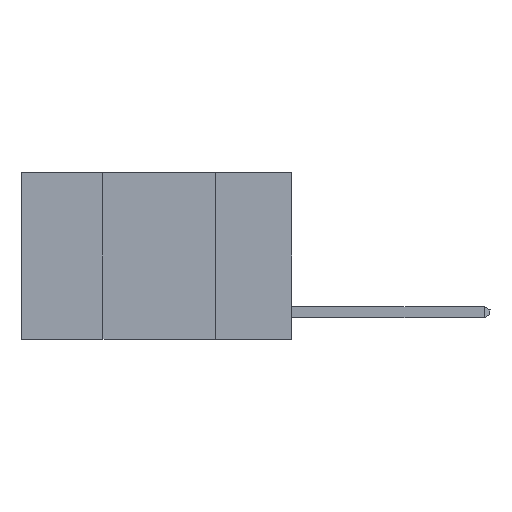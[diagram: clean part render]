
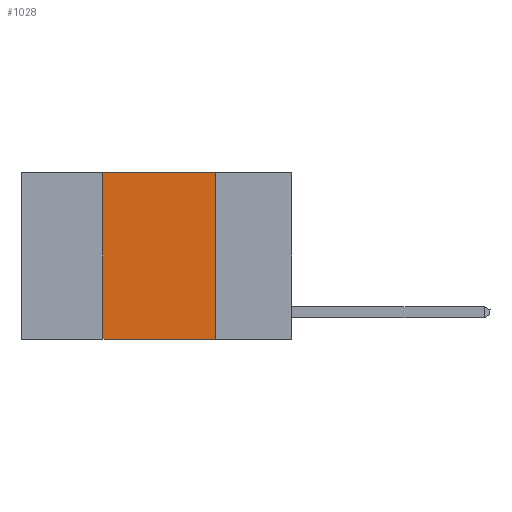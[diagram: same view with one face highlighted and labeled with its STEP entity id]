
A CAD part, left-side view. The second image highlights one B-rep face of the part: STEP entity #1028.
In plain terms, the highlighted planar face has unit normal (-1, 0, 0).
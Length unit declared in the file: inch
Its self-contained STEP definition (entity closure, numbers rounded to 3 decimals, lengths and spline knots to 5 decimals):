
#1028 = ADVANCED_FACE ( 'NONE', ( #15249 ), #13510, .F. ) ;
#2885 = CARTESIAN_POINT ( 'NONE',  ( 0., 0.17, 0. ) ) ;
#3431 = LINE ( 'NONE', #13747, #8251 ) ;
#3670 = VERTEX_POINT ( 'NONE', #6713 ) ;
#4139 = EDGE_CURVE ( 'NONE', #3670, #15752, #3431, .T. ) ;
#4483 = ORIENTED_EDGE ( 'NONE', *, *, #4139, .F. ) ;
#5009 = VECTOR ( 'NONE', #19134, 39.37008 ) ;
#6699 = CARTESIAN_POINT ( 'NONE',  ( 0., 0.6, -0.37 ) ) ;
#6713 = CARTESIAN_POINT ( 'NONE',  ( 0., 0.42, 0. ) ) ;
#7006 = ORIENTED_EDGE ( 'NONE', *, *, #11536, .T. ) ;
#7026 = LINE ( 'NONE', #15766, #8327 ) ;
#8251 = VECTOR ( 'NONE', #26389, 39.37008 ) ;
#8327 = VECTOR ( 'NONE', #21846, 39.37008 ) ;
#8535 = VECTOR ( 'NONE', #25374, 39.37008 ) ;
#10276 = VERTEX_POINT ( 'NONE', #21346 ) ;
#11498 = LINE ( 'NONE', #6699, #5009 ) ;
#11536 = EDGE_CURVE ( 'NONE', #10276, #22164, #11498, .T. ) ;
#11860 = EDGE_CURVE ( 'NONE', #15752, #22164, #19908, .T. ) ;
#13510 = PLANE ( 'NONE',  #16265 ) ;
#13747 = CARTESIAN_POINT ( 'NONE',  ( 0., 0.6, 0. ) ) ;
#14079 = DIRECTION ( 'NONE',  ( 0., 0., -1. ) ) ;
#14887 = CARTESIAN_POINT ( 'NONE',  ( 0., 0.17, -0.37 ) ) ;
#15249 = FACE_OUTER_BOUND ( 'NONE', #20489, .T. ) ;
#15752 = VERTEX_POINT ( 'NONE', #22078 ) ;
#15766 = CARTESIAN_POINT ( 'NONE',  ( 0., 0.42, 0. ) ) ;
#16265 = AXIS2_PLACEMENT_3D ( 'NONE', #19367, #24610, #14079 ) ;
#19134 = DIRECTION ( 'NONE',  ( 0., -1., 0. ) ) ;
#19367 = CARTESIAN_POINT ( 'NONE',  ( 0., 0.6, 0. ) ) ;
#19532 = ORIENTED_EDGE ( 'NONE', *, *, #26496, .F. ) ;
#19908 = LINE ( 'NONE', #2885, #8535 ) ;
#20489 = EDGE_LOOP ( 'NONE', ( #20653, #4483, #19532, #7006 ) ) ;
#20653 = ORIENTED_EDGE ( 'NONE', *, *, #11860, .F. ) ;
#21346 = CARTESIAN_POINT ( 'NONE',  ( 0., 0.42, -0.37 ) ) ;
#21846 = DIRECTION ( 'NONE',  ( 0., 0., 1. ) ) ;
#22078 = CARTESIAN_POINT ( 'NONE',  ( 0., 0.17, 0. ) ) ;
#22164 = VERTEX_POINT ( 'NONE', #14887 ) ;
#24610 = DIRECTION ( 'NONE',  ( 1., 0., 0. ) ) ;
#25374 = DIRECTION ( 'NONE',  ( 0., 0., -1. ) ) ;
#26389 = DIRECTION ( 'NONE',  ( 0., -1., 0. ) ) ;
#26496 = EDGE_CURVE ( 'NONE', #10276, #3670, #7026, .T. ) ;
